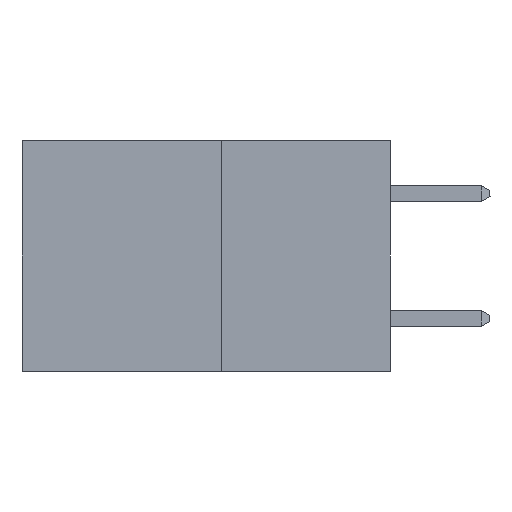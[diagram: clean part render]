
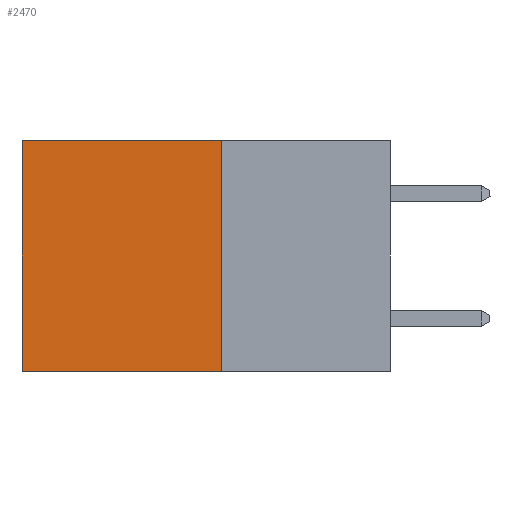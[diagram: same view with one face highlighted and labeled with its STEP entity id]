
A CAD part, left-side view. The second image highlights one B-rep face of the part: STEP entity #2470.
In plain terms, the highlighted planar face has unit normal (-1, 0, 0).
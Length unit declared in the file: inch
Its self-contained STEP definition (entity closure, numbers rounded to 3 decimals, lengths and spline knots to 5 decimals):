
#105 = CARTESIAN_POINT ( 'NONE',  ( 0.277, 0.27, -0.37 ) ) ;
#249 = EDGE_CURVE ( 'NONE', #9506, #4455, #2941, .T. ) ;
#829 = VERTEX_POINT ( 'NONE', #8167 ) ;
#1071 = LINE ( 'NONE', #2797, #5311 ) ;
#1169 = LINE ( 'NONE', #1476, #3140 ) ;
#1273 = ORIENTED_EDGE ( 'NONE', *, *, #8080, .T. ) ;
#1426 = ORIENTED_EDGE ( 'NONE', *, *, #5958, .F. ) ;
#1476 = CARTESIAN_POINT ( 'NONE',  ( 0.277, 0.59, -0.37 ) ) ;
#1494 = EDGE_CURVE ( 'NONE', #9506, #829, #5913, .T. ) ;
#1740 = AXIS2_PLACEMENT_3D ( 'NONE', #5030, #4858, #4828 ) ;
#2075 = ORIENTED_EDGE ( 'NONE', *, *, #1494, .F. ) ;
#2470 = ADVANCED_FACE ( 'NONE', ( #3406 ), #5271, .F. ) ;
#2797 = CARTESIAN_POINT ( 'NONE',  ( 0.277, 0.27, -0.37 ) ) ;
#2941 = LINE ( 'NONE', #3542, #5211 ) ;
#3031 = CARTESIAN_POINT ( 'NONE',  ( 0.277, 0.59, -0.37 ) ) ;
#3140 = VECTOR ( 'NONE', #3786, 39.37008 ) ;
#3303 = DIRECTION ( 'NONE',  ( 0., 1., 0. ) ) ;
#3406 = FACE_OUTER_BOUND ( 'NONE', #4093, .T. ) ;
#3542 = CARTESIAN_POINT ( 'NONE',  ( 0.277, 0.27, 0. ) ) ;
#3786 = DIRECTION ( 'NONE',  ( 0., 0., -1. ) ) ;
#3827 = ORIENTED_EDGE ( 'NONE', *, *, #249, .T. ) ;
#3890 = VECTOR ( 'NONE', #9932, 39.37008 ) ;
#4093 = EDGE_LOOP ( 'NONE', ( #1273, #1426, #2075, #3827 ) ) ;
#4366 = VERTEX_POINT ( 'NONE', #3031 ) ;
#4455 = VERTEX_POINT ( 'NONE', #6821 ) ;
#4828 = DIRECTION ( 'NONE',  ( 0., 0., -1. ) ) ;
#4858 = DIRECTION ( 'NONE',  ( 1., 0., 0. ) ) ;
#5030 = CARTESIAN_POINT ( 'NONE',  ( 0.277, 0.27, -0.37 ) ) ;
#5211 = VECTOR ( 'NONE', #3303, 39.37008 ) ;
#5271 = PLANE ( 'NONE',  #1740 ) ;
#5311 = VECTOR ( 'NONE', #6551, 39.37008 ) ;
#5913 = LINE ( 'NONE', #105, #3890 ) ;
#5958 = EDGE_CURVE ( 'NONE', #829, #4366, #1071, .T. ) ;
#6551 = DIRECTION ( 'NONE',  ( 0., 1., 0. ) ) ;
#6637 = CARTESIAN_POINT ( 'NONE',  ( 0.277, 0.27, 0. ) ) ;
#6821 = CARTESIAN_POINT ( 'NONE',  ( 0.277, 0.59, 0. ) ) ;
#8080 = EDGE_CURVE ( 'NONE', #4455, #4366, #1169, .T. ) ;
#8167 = CARTESIAN_POINT ( 'NONE',  ( 0.277, 0.27, -0.37 ) ) ;
#9506 = VERTEX_POINT ( 'NONE', #6637 ) ;
#9932 = DIRECTION ( 'NONE',  ( 0., 0., -1. ) ) ;
